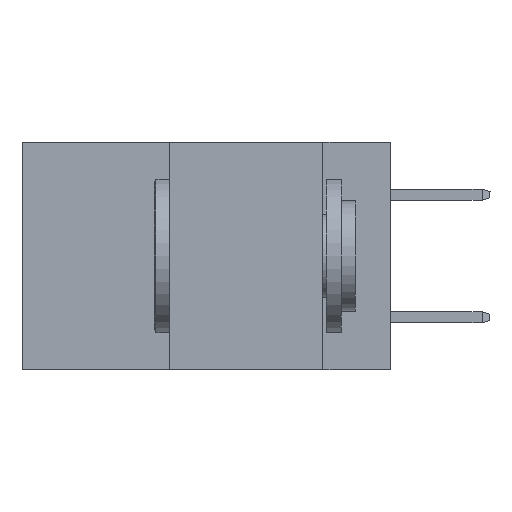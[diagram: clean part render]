
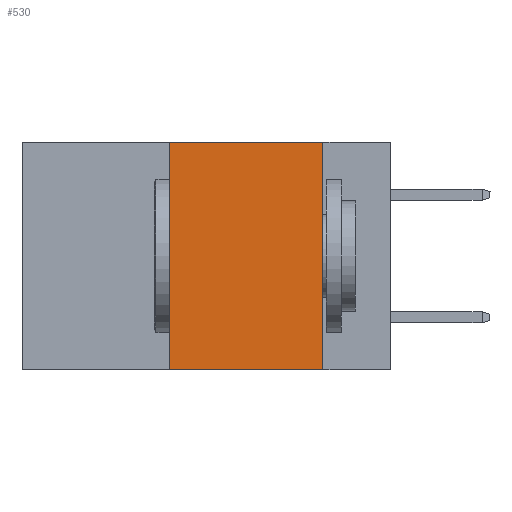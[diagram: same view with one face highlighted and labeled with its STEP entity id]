
A CAD part, left-side view. The second image highlights one B-rep face of the part: STEP entity #530.
In plain terms, the highlighted planar face has unit normal (-1, 0, 0).
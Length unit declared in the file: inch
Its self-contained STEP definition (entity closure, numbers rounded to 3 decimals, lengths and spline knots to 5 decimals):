
#530 = ADVANCED_FACE ( 'NONE', ( #8482 ), #1243, .F. ) ;
#626 = EDGE_CURVE ( 'NONE', #11304, #6303, #5782, .T. ) ;
#811 = VERTEX_POINT ( 'NONE', #3764 ) ;
#1243 = PLANE ( 'NONE',  #2100 ) ;
#1322 = CARTESIAN_POINT ( 'NONE',  ( 0., 0.6, 0. ) ) ;
#1606 = EDGE_CURVE ( 'NONE', #7393, #811, #2388, .T. ) ;
#2033 = EDGE_LOOP ( 'NONE', ( #4965, #9548, #9067, #8417 ) ) ;
#2099 = VECTOR ( 'NONE', #6856, 39.37008 ) ;
#2100 = AXIS2_PLACEMENT_3D ( 'NONE', #8551, #9454, #10369 ) ;
#2388 = LINE ( 'NONE', #1322, #2099 ) ;
#3451 = EDGE_CURVE ( 'NONE', #811, #6303, #11129, .T. ) ;
#3591 = CARTESIAN_POINT ( 'NONE',  ( 0., 0.36, 0. ) ) ;
#3626 = DIRECTION ( 'NONE',  ( 0., 0., 1. ) ) ;
#3764 = CARTESIAN_POINT ( 'NONE',  ( 0., 0.11, 0. ) ) ;
#4055 = CARTESIAN_POINT ( 'NONE',  ( 0., 0.11, 0. ) ) ;
#4161 = CARTESIAN_POINT ( 'NONE',  ( 0., 0.6, -0.37 ) ) ;
#4350 = VECTOR ( 'NONE', #3626, 39.37008 ) ;
#4362 = CARTESIAN_POINT ( 'NONE',  ( 0., 0.36, -0.37 ) ) ;
#4965 = ORIENTED_EDGE ( 'NONE', *, *, #3451, .F. ) ;
#5782 = LINE ( 'NONE', #4161, #6948 ) ;
#6303 = VERTEX_POINT ( 'NONE', #6582 ) ;
#6582 = CARTESIAN_POINT ( 'NONE',  ( 0., 0.11, -0.37 ) ) ;
#6856 = DIRECTION ( 'NONE',  ( 0., -1., 0. ) ) ;
#6948 = VECTOR ( 'NONE', #9777, 39.37008 ) ;
#7204 = LINE ( 'NONE', #3591, #4350 ) ;
#7393 = VERTEX_POINT ( 'NONE', #8407 ) ;
#7448 = VECTOR ( 'NONE', #10416, 39.37008 ) ;
#8407 = CARTESIAN_POINT ( 'NONE',  ( 0., 0.36, 0. ) ) ;
#8417 = ORIENTED_EDGE ( 'NONE', *, *, #626, .T. ) ;
#8482 = FACE_OUTER_BOUND ( 'NONE', #2033, .T. ) ;
#8551 = CARTESIAN_POINT ( 'NONE',  ( 0., 0.6, 0. ) ) ;
#9067 = ORIENTED_EDGE ( 'NONE', *, *, #9414, .F. ) ;
#9414 = EDGE_CURVE ( 'NONE', #11304, #7393, #7204, .T. ) ;
#9454 = DIRECTION ( 'NONE',  ( 1., 0., 0. ) ) ;
#9548 = ORIENTED_EDGE ( 'NONE', *, *, #1606, .F. ) ;
#9777 = DIRECTION ( 'NONE',  ( 0., -1., 0. ) ) ;
#10369 = DIRECTION ( 'NONE',  ( 0., 0., -1. ) ) ;
#10416 = DIRECTION ( 'NONE',  ( 0., 0., -1. ) ) ;
#11129 = LINE ( 'NONE', #4055, #7448 ) ;
#11304 = VERTEX_POINT ( 'NONE', #4362 ) ;
